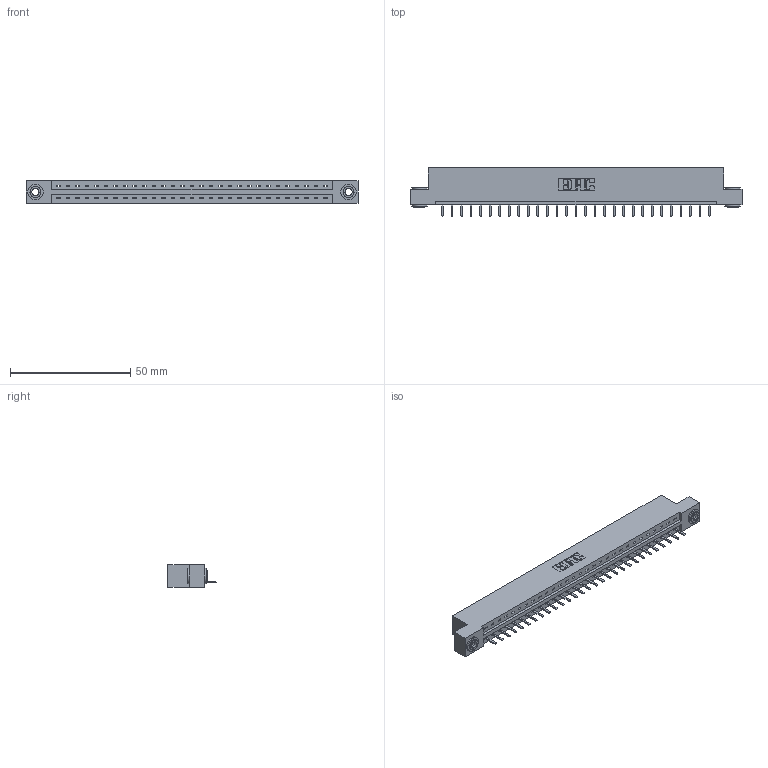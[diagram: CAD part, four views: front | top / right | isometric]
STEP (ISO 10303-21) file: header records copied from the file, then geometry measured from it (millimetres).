
FILE_DESCRIPTION (( 'STEP AP203' ), '1' );
FILE_NAME ('387-029-520-103.STEP', '2018-09-17T00:48:40', ( '' ), ( '' ), 'SwSTEP 2.0', 'SolidWorks 2016', '' );
FILE_SCHEMA (( 'CONFIG_CONTROL_DESIGN' ));
Length unit declared in the file: inch
Products named in the file (4): 337 Part_Flush Mounting Lugs - 0.156 Dia-TH; 345-292-001_345-293-120; 345-250-002_345-250-002-102; 387-029-520-103
Assembly tree (32 placements, depth 2):
  387-029-520-103
    337 Part_Flush Mounting Lugs - 0.156 Dia-TH
    345-292-001_345-293-120  x29
    345-250-002_345-250-002-102  x2
Bounding box: 137.92 x 20.02 x 9.4 mm (x, y, z)
Volume: 14108 mm3; surface area: 14438.8 mm2
Topology: 32 solids, 32 shells, 2066 faces, 6071 edges, 3966 vertices
Faces by surface type: plane 1472, cylinder 586, cone 8
Entity records: 24002 total; most frequent: CARTESIAN_POINT 4168, ORIENTED_EDGE 4114, DIRECTION 3557, EDGE_CURVE 2057, VECTOR 1901, LINE 1901, VERTEX_POINT 1366, AXIS2_PLACEMENT_3D 828
